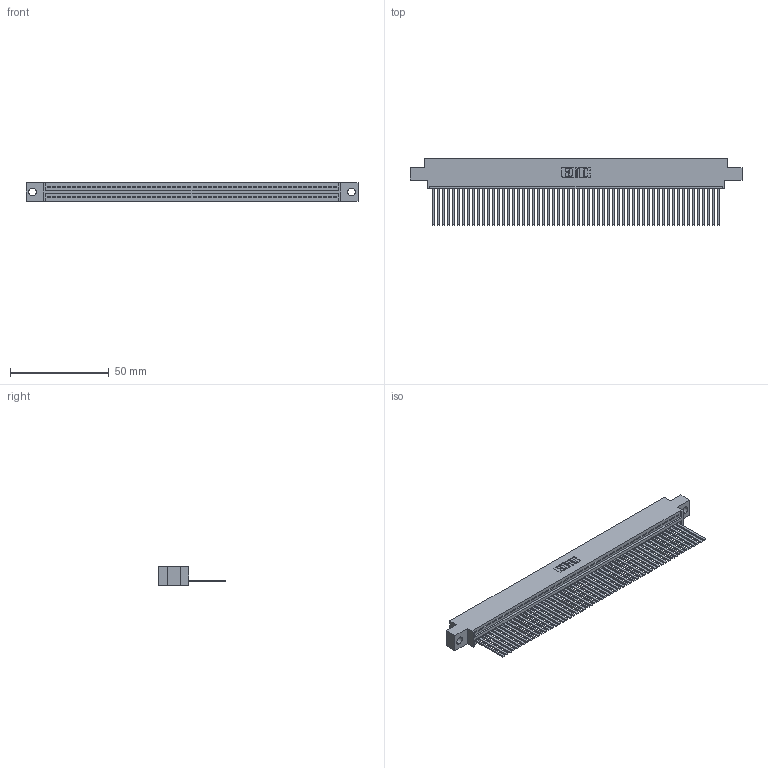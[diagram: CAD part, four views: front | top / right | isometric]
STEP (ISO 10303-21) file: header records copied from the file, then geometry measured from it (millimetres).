
FILE_DESCRIPTION (( 'STEP AP203' ), '1' );
FILE_NAME ('345-058-544-604.STEP', '2018-09-26T16:09:01', ( '' ), ( '' ), 'SwSTEP 2.0', 'SolidWorks 2016', '' );
FILE_SCHEMA (( 'CONFIG_CONTROL_DESIGN' ));
Length unit declared in the file: inch
Products named in the file (3): 345-292-001_345-293-144; 345-058-544-604; 345 Part_0.170 Offset - 0.156 Dia-TH
Assembly tree (59 placements, depth 2):
  345-058-544-604
    345 Part_0.170 Offset - 0.156 Dia-TH
    345-292-001_345-293-144  x58
Bounding box: 168.53 x 33.96 x 9.4 mm (x, y, z)
Volume: 16608.6 mm3; surface area: 24240.7 mm2
Topology: 59 solids, 59 shells, 3146 faces, 9517 edges, 6266 vertices
Faces by surface type: plane 2172, cylinder 974
Entity records: 41449 total; most frequent: CARTESIAN_POINT 7186, ORIENTED_EDGE 7178, DIRECTION 6249, EDGE_CURVE 3589, VECTOR 3229, LINE 3229, VERTEX_POINT 2390, AXIS2_PLACEMENT_3D 1510
